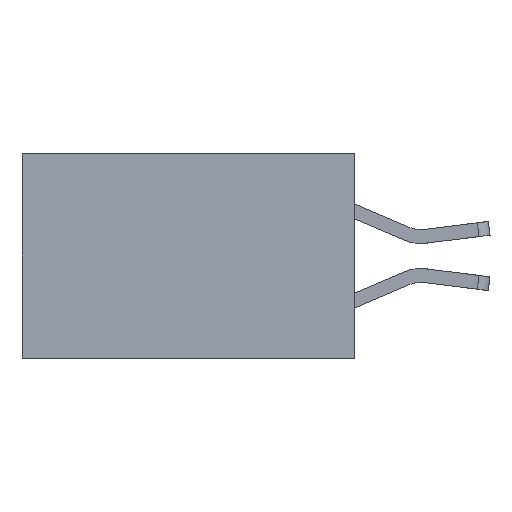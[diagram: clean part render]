
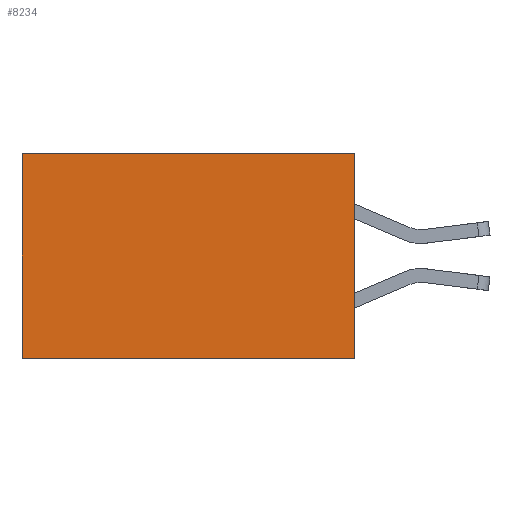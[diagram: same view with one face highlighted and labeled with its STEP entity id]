
A CAD part, left-side view. The second image highlights one B-rep face of the part: STEP entity #8234.
In plain terms, the highlighted planar face has unit normal (-1, 0, 0).
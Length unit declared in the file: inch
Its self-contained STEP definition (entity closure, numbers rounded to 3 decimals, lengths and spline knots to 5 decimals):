
#542 = VECTOR ( 'NONE', #10547, 39.37008 ) ;
#1127 = ORIENTED_EDGE ( 'NONE', *, *, #3664, .F. ) ;
#1959 = VERTEX_POINT ( 'NONE', #2145 ) ;
#2021 = PLANE ( 'NONE',  #8985 ) ;
#2047 = EDGE_CURVE ( 'NONE', #11312, #1959, #2380, .T. ) ;
#2053 = VECTOR ( 'NONE', #7410, 39.37008 ) ;
#2145 = CARTESIAN_POINT ( 'NONE',  ( 0.298, 0.6, -0.37 ) ) ;
#2380 = LINE ( 'NONE', #10774, #2053 ) ;
#3042 = CARTESIAN_POINT ( 'NONE',  ( 0.298, 0., 0. ) ) ;
#3102 = VERTEX_POINT ( 'NONE', #5795 ) ;
#3159 = DIRECTION ( 'NONE',  ( 0., 1., 0. ) ) ;
#3664 = EDGE_CURVE ( 'NONE', #3102, #1959, #5898, .T. ) ;
#3859 = VECTOR ( 'NONE', #9168, 39.37008 ) ;
#4006 = DIRECTION ( 'NONE',  ( 0., 0., -1. ) ) ;
#5663 = VERTEX_POINT ( 'NONE', #6402 ) ;
#5795 = CARTESIAN_POINT ( 'NONE',  ( 0.298, 0., -0.37 ) ) ;
#5898 = LINE ( 'NONE', #9777, #8263 ) ;
#6402 = CARTESIAN_POINT ( 'NONE',  ( 0.298, 0., 0. ) ) ;
#7383 = CARTESIAN_POINT ( 'NONE',  ( 0.298, 0., 0. ) ) ;
#7410 = DIRECTION ( 'NONE',  ( 0., 0., -1. ) ) ;
#7525 = EDGE_CURVE ( 'NONE', #5663, #11312, #11056, .T. ) ;
#8234 = ADVANCED_FACE ( 'NONE', ( #9775 ), #2021, .F. ) ;
#8263 = VECTOR ( 'NONE', #3159, 39.37008 ) ;
#8624 = EDGE_LOOP ( 'NONE', ( #8626, #1127, #11579, #11765 ) ) ;
#8626 = ORIENTED_EDGE ( 'NONE', *, *, #2047, .T. ) ;
#8985 = AXIS2_PLACEMENT_3D ( 'NONE', #3042, #9392, #4006 ) ;
#9111 = CARTESIAN_POINT ( 'NONE',  ( 0.298, 0.6, 0. ) ) ;
#9168 = DIRECTION ( 'NONE',  ( 0., 1., 0. ) ) ;
#9392 = DIRECTION ( 'NONE',  ( 1., 0., 0. ) ) ;
#9775 = FACE_OUTER_BOUND ( 'NONE', #8624, .T. ) ;
#9777 = CARTESIAN_POINT ( 'NONE',  ( 0.298, 0., -0.37 ) ) ;
#10294 = EDGE_CURVE ( 'NONE', #5663, #3102, #10465, .T. ) ;
#10465 = LINE ( 'NONE', #11411, #542 ) ;
#10547 = DIRECTION ( 'NONE',  ( 0., 0., -1. ) ) ;
#10774 = CARTESIAN_POINT ( 'NONE',  ( 0.298, 0.6, 0. ) ) ;
#11056 = LINE ( 'NONE', #7383, #3859 ) ;
#11312 = VERTEX_POINT ( 'NONE', #9111 ) ;
#11411 = CARTESIAN_POINT ( 'NONE',  ( 0.298, 0., 0. ) ) ;
#11579 = ORIENTED_EDGE ( 'NONE', *, *, #10294, .F. ) ;
#11765 = ORIENTED_EDGE ( 'NONE', *, *, #7525, .T. ) ;
